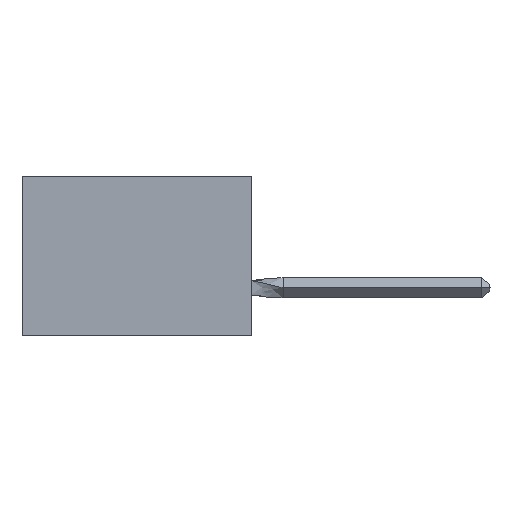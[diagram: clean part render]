
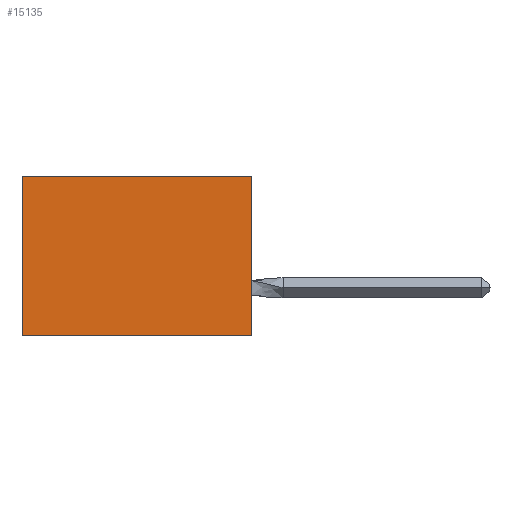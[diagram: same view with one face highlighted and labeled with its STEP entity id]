
A CAD part, left-side view. The second image highlights one B-rep face of the part: STEP entity #15135.
In plain terms, the highlighted planar face has unit normal (-1, 0, 0).
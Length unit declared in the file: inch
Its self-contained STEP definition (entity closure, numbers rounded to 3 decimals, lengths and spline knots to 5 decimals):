
#1105 = VECTOR ( 'NONE', #24980, 39.37008 ) ;
#1683 = CARTESIAN_POINT ( 'NONE',  ( 0.305, 0.72, -0.5 ) ) ;
#1689 = VERTEX_POINT ( 'NONE', #10833 ) ;
#3993 = EDGE_CURVE ( 'NONE', #29022, #24295, #19822, .T. ) ;
#4450 = DIRECTION ( 'NONE',  ( 1., 0., 0. ) ) ;
#5759 = CARTESIAN_POINT ( 'NONE',  ( 0.305, 0.72, -0.5 ) ) ;
#6599 = DIRECTION ( 'NONE',  ( 0., 0., -1. ) ) ;
#6601 = VECTOR ( 'NONE', #8160, 39.37008 ) ;
#6690 = ORIENTED_EDGE ( 'NONE', *, *, #3993, .T. ) ;
#7072 = EDGE_CURVE ( 'NONE', #11322, #29022, #14352, .T. ) ;
#8160 = DIRECTION ( 'NONE',  ( 0., 1., 0. ) ) ;
#9659 = ORIENTED_EDGE ( 'NONE', *, *, #25829, .F. ) ;
#9684 = LINE ( 'NONE', #20012, #1105 ) ;
#10833 = CARTESIAN_POINT ( 'NONE',  ( 0.305, 0., -0.5 ) ) ;
#11322 = VERTEX_POINT ( 'NONE', #15386 ) ;
#13071 = AXIS2_PLACEMENT_3D ( 'NONE', #19592, #4450, #6599 ) ;
#14352 = LINE ( 'NONE', #18404, #6601 ) ;
#15135 = ADVANCED_FACE ( 'NONE', ( #19023 ), #20044, .F. ) ;
#15386 = CARTESIAN_POINT ( 'NONE',  ( 0.305, 0., 0. ) ) ;
#16448 = LINE ( 'NONE', #17140, #25403 ) ;
#17140 = CARTESIAN_POINT ( 'NONE',  ( 0.305, 0., -0.5 ) ) ;
#17742 = ORIENTED_EDGE ( 'NONE', *, *, #24251, .F. ) ;
#18404 = CARTESIAN_POINT ( 'NONE',  ( 0.305, 0., 0. ) ) ;
#19023 = FACE_OUTER_BOUND ( 'NONE', #30391, .T. ) ;
#19592 = CARTESIAN_POINT ( 'NONE',  ( 0.305, 0., -0.5 ) ) ;
#19822 = LINE ( 'NONE', #5759, #25500 ) ;
#20012 = CARTESIAN_POINT ( 'NONE',  ( 0.305, 0., -0.5 ) ) ;
#20044 = PLANE ( 'NONE',  #13071 ) ;
#20119 = DIRECTION ( 'NONE',  ( 0., 0., -1. ) ) ;
#20126 = ORIENTED_EDGE ( 'NONE', *, *, #7072, .T. ) ;
#21729 = CARTESIAN_POINT ( 'NONE',  ( 0.305, 0.72, 0. ) ) ;
#24061 = DIRECTION ( 'NONE',  ( 0., 0., -1. ) ) ;
#24251 = EDGE_CURVE ( 'NONE', #1689, #24295, #9684, .T. ) ;
#24295 = VERTEX_POINT ( 'NONE', #1683 ) ;
#24980 = DIRECTION ( 'NONE',  ( 0., 1., 0. ) ) ;
#25403 = VECTOR ( 'NONE', #20119, 39.37008 ) ;
#25500 = VECTOR ( 'NONE', #24061, 39.37008 ) ;
#25829 = EDGE_CURVE ( 'NONE', #11322, #1689, #16448, .T. ) ;
#29022 = VERTEX_POINT ( 'NONE', #21729 ) ;
#30391 = EDGE_LOOP ( 'NONE', ( #6690, #17742, #9659, #20126 ) ) ;
